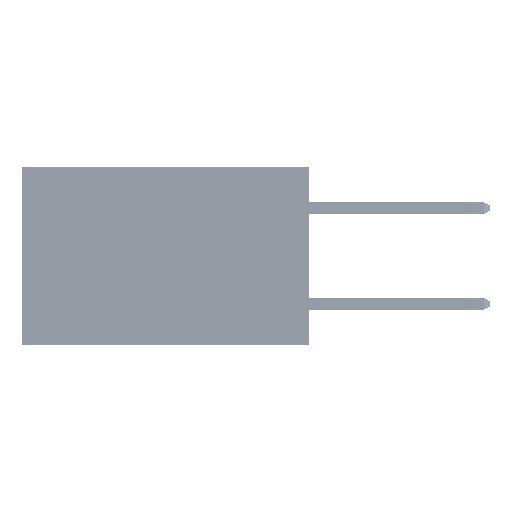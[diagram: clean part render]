
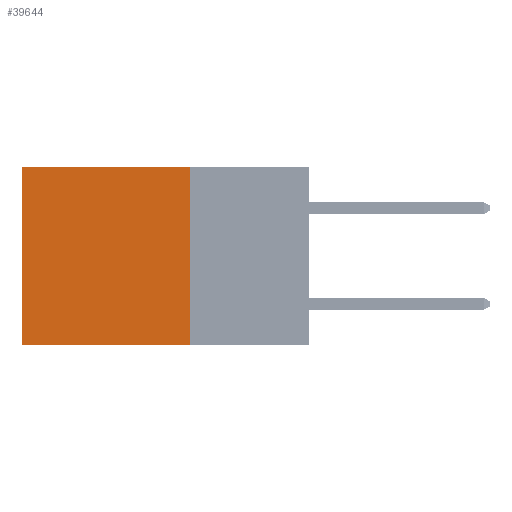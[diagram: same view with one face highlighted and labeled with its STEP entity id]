
A CAD part, left-side view. The second image highlights one B-rep face of the part: STEP entity #39644.
In plain terms, the highlighted planar face has unit normal (-1, 0, 0).
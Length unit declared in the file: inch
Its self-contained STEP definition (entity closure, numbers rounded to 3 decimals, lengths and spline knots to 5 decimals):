
#467 = CARTESIAN_POINT ( 'NONE',  ( 0.2875, 0.6, 0. ) ) ;
#1628 = EDGE_CURVE ( 'NONE', #20948, #30853, #41100, .T. ) ;
#4363 = FACE_OUTER_BOUND ( 'NONE', #28889, .T. ) ;
#6562 = CARTESIAN_POINT ( 'NONE',  ( 0.2875, 0.25, 0. ) ) ;
#11098 = EDGE_CURVE ( 'NONE', #30853, #23638, #34429, .T. ) ;
#13496 = VECTOR ( 'NONE', #30190, 39.37008 ) ;
#15851 = VECTOR ( 'NONE', #30507, 39.37008 ) ;
#18984 = DIRECTION ( 'NONE',  ( 0., 0., -1. ) ) ;
#20948 = VERTEX_POINT ( 'NONE', #35436 ) ;
#21568 = VECTOR ( 'NONE', #34811, 39.37008 ) ;
#22192 = EDGE_CURVE ( 'NONE', #20948, #33564, #28532, .T. ) ;
#23557 = PLANE ( 'NONE',  #36310 ) ;
#23638 = VERTEX_POINT ( 'NONE', #48615 ) ;
#24149 = CARTESIAN_POINT ( 'NONE',  ( 0.2875, 0.25, -0.37 ) ) ;
#28532 = LINE ( 'NONE', #30779, #21568 ) ;
#28889 = EDGE_LOOP ( 'NONE', ( #39527, #51321, #52333, #40202 ) ) ;
#30190 = DIRECTION ( 'NONE',  ( 0., 0., -1. ) ) ;
#30507 = DIRECTION ( 'NONE',  ( 0., 0., -1. ) ) ;
#30534 = CARTESIAN_POINT ( 'NONE',  ( 0.2875, 0.6, 0. ) ) ;
#30779 = CARTESIAN_POINT ( 'NONE',  ( 0.2875, 0.25, 0. ) ) ;
#30853 = VERTEX_POINT ( 'NONE', #24149 ) ;
#33564 = VERTEX_POINT ( 'NONE', #467 ) ;
#34429 = LINE ( 'NONE', #51500, #49634 ) ;
#34811 = DIRECTION ( 'NONE',  ( 0., 1., 0. ) ) ;
#34963 = LINE ( 'NONE', #30534, #13496 ) ;
#35436 = CARTESIAN_POINT ( 'NONE',  ( 0.2875, 0.25, 0. ) ) ;
#36310 = AXIS2_PLACEMENT_3D ( 'NONE', #6562, #47229, #18984 ) ;
#39527 = ORIENTED_EDGE ( 'NONE', *, *, #46604, .T. ) ;
#39644 = ADVANCED_FACE ( 'NONE', ( #4363 ), #23557, .F. ) ;
#40202 = ORIENTED_EDGE ( 'NONE', *, *, #22192, .T. ) ;
#41100 = LINE ( 'NONE', #51017, #15851 ) ;
#44606 = DIRECTION ( 'NONE',  ( 0., 1., 0. ) ) ;
#46604 = EDGE_CURVE ( 'NONE', #33564, #23638, #34963, .T. ) ;
#47229 = DIRECTION ( 'NONE',  ( 1., 0., 0. ) ) ;
#48615 = CARTESIAN_POINT ( 'NONE',  ( 0.2875, 0.6, -0.37 ) ) ;
#49634 = VECTOR ( 'NONE', #44606, 39.37008 ) ;
#51017 = CARTESIAN_POINT ( 'NONE',  ( 0.2875, 0.25, 0. ) ) ;
#51321 = ORIENTED_EDGE ( 'NONE', *, *, #11098, .F. ) ;
#51500 = CARTESIAN_POINT ( 'NONE',  ( 0.2875, 0.25, -0.37 ) ) ;
#52333 = ORIENTED_EDGE ( 'NONE', *, *, #1628, .F. ) ;
